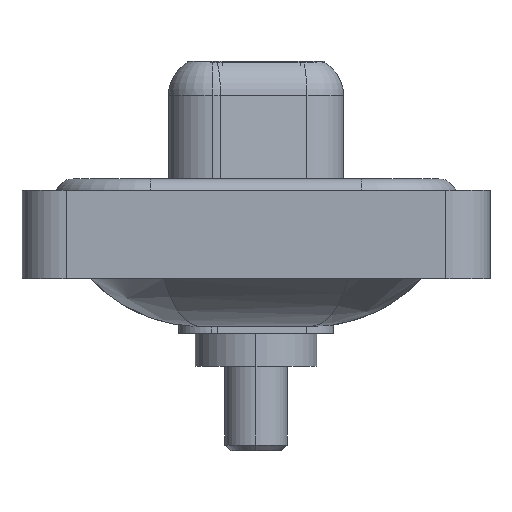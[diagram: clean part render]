
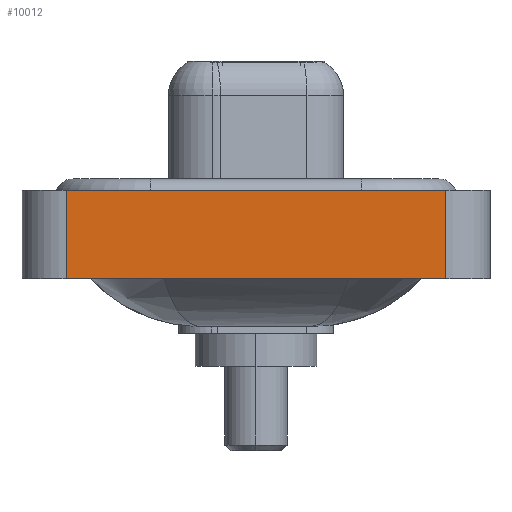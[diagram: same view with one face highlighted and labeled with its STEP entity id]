
A CAD part, left-side view. The second image highlights one B-rep face of the part: STEP entity #10012.
In plain terms, the highlighted planar face has unit normal (-1, 0, 0).
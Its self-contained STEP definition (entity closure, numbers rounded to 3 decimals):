
#424 = CARTESIAN_POINT ( 'NONE',  ( -7.3, 8.55, -3.6 ) ) ;
#513 = DIRECTION ( 'NONE',  ( 0., 0., 1. ) ) ;
#589 = ORIENTED_EDGE ( 'NONE', *, *, #3651, .F. ) ;
#761 = FACE_OUTER_BOUND ( 'NONE', #8150, .T. ) ;
#2124 = DIRECTION ( 'NONE',  ( 0., -1., 0. ) ) ;
#2263 = ORIENTED_EDGE ( 'NONE', *, *, #13283, .T. ) ;
#2524 = CARTESIAN_POINT ( 'NONE',  ( -7.3, -8.55, -3.6 ) ) ;
#2801 = VECTOR ( 'NONE', #513, 1000. ) ;
#3270 = LINE ( 'NONE', #7255, #8759 ) ;
#3417 = VECTOR ( 'NONE', #15011, 1000. ) ;
#3651 = EDGE_CURVE ( 'NONE', #11784, #16354, #4140, .T. ) ;
#4062 = ORIENTED_EDGE ( 'NONE', *, *, #14557, .F. ) ;
#4132 = CARTESIAN_POINT ( 'NONE',  ( -7.3, -8.55, -3.6 ) ) ;
#4140 = LINE ( 'NONE', #7883, #2801 ) ;
#5202 = DIRECTION ( 'NONE',  ( 0., -1., 0. ) ) ;
#5894 = CARTESIAN_POINT ( 'NONE',  ( -7.3, -8.55, -3.6 ) ) ;
#6167 = DIRECTION ( 'NONE',  ( -1., 0., 0. ) ) ;
#6274 = CARTESIAN_POINT ( 'NONE',  ( -7.3, -8.55, -3.6 ) ) ;
#6905 = VERTEX_POINT ( 'NONE', #11271 ) ;
#7255 = CARTESIAN_POINT ( 'NONE',  ( -7.3, -8.55, 0.4 ) ) ;
#7883 = CARTESIAN_POINT ( 'NONE',  ( -7.3, 8.55, -3.6 ) ) ;
#8150 = EDGE_LOOP ( 'NONE', ( #2263, #4062, #589, #9699 ) ) ;
#8759 = VECTOR ( 'NONE', #2124, 1000. ) ;
#9699 = ORIENTED_EDGE ( 'NONE', *, *, #15405, .T. ) ;
#9841 = VERTEX_POINT ( 'NONE', #5894 ) ;
#10012 = ADVANCED_FACE ( 'NONE', ( #761 ), #14493, .T. ) ;
#10859 = LINE ( 'NONE', #4132, #12174 ) ;
#11271 = CARTESIAN_POINT ( 'NONE',  ( -7.3, -8.55, 0.4 ) ) ;
#11784 = VERTEX_POINT ( 'NONE', #424 ) ;
#12174 = VECTOR ( 'NONE', #5202, 1000. ) ;
#12258 = LINE ( 'NONE', #2524, #3417 ) ;
#13283 = EDGE_CURVE ( 'NONE', #9841, #6905, #12258, .T. ) ;
#14228 = DIRECTION ( 'NONE',  ( 0., 0., 1. ) ) ;
#14493 = PLANE ( 'NONE',  #15039 ) ;
#14557 = EDGE_CURVE ( 'NONE', #16354, #6905, #3270, .T. ) ;
#15011 = DIRECTION ( 'NONE',  ( 0., 0., 1. ) ) ;
#15039 = AXIS2_PLACEMENT_3D ( 'NONE', #6274, #6167, #14228 ) ;
#15405 = EDGE_CURVE ( 'NONE', #11784, #9841, #10859, .T. ) ;
#16354 = VERTEX_POINT ( 'NONE', #17315 ) ;
#17315 = CARTESIAN_POINT ( 'NONE',  ( -7.3, 8.55, 0.4 ) ) ;
